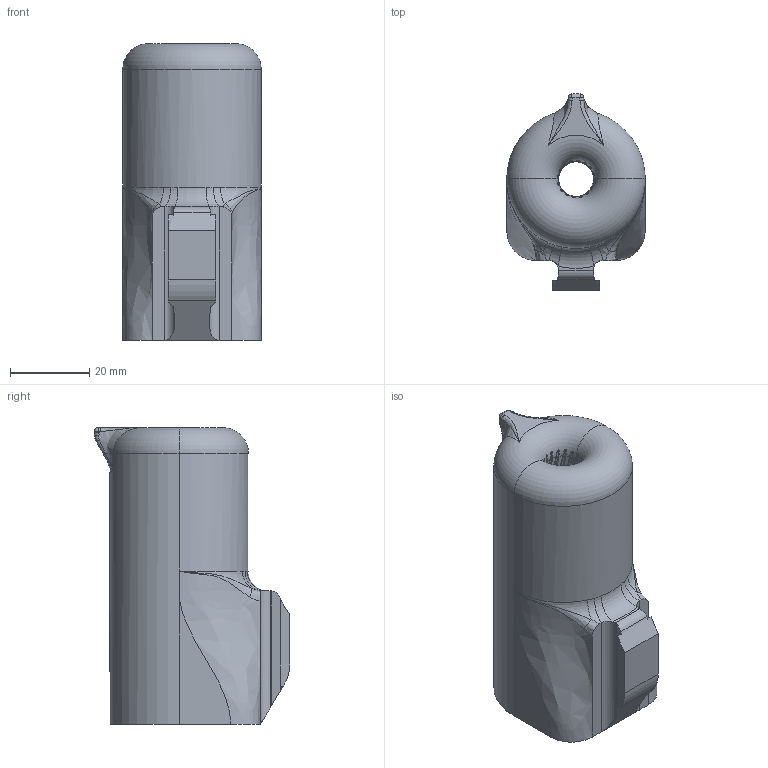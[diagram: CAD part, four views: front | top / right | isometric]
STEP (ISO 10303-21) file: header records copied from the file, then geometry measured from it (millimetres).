
FILE_DESCRIPTION (( 'STEP AP214' ), '1' );
FILE_NAME ('Barrel_Long.STEP', '2014-02-22T02:08:09', ( '' ), ( '' ), 'SwSTEP 2.0', 'SolidWorks 2013', '' );
FILE_SCHEMA (( 'AUTOMOTIVE_DESIGN' ));
Length unit declared in the file: millimetre
Products named in the file (1): Barrel_Long
Bounding box: 35 x 49.5 x 75 mm (x, y, z)
Volume: 73144.5 mm3; surface area: 13346 mm2
Topology: 1 solids, 1 shells, 182 faces, 461 edges, 276 vertices
Faces by surface type: bspline 90, cylinder 41, plane 40, torus 8, sphere 2, cone 1
Entity records: 14273 total; most frequent: CARTESIAN_POINT 10541, ORIENTED_EDGE 914, DIRECTION 613, EDGE_CURVE 457, VERTEX_POINT 276, AXIS2_PLACEMENT_3D 268, B_SPLINE_CURVE_WITH_KNOTS 195, EDGE_LOOP 183
